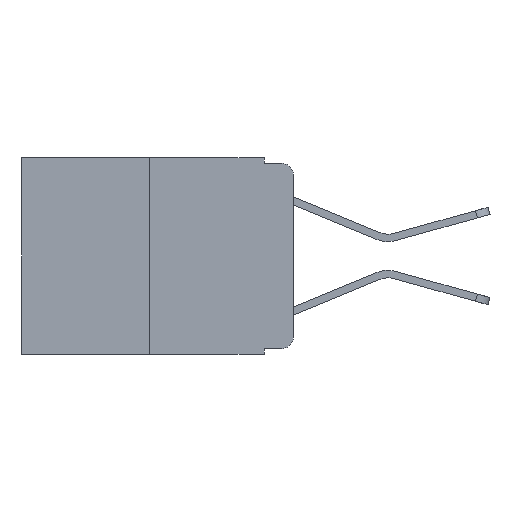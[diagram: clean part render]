
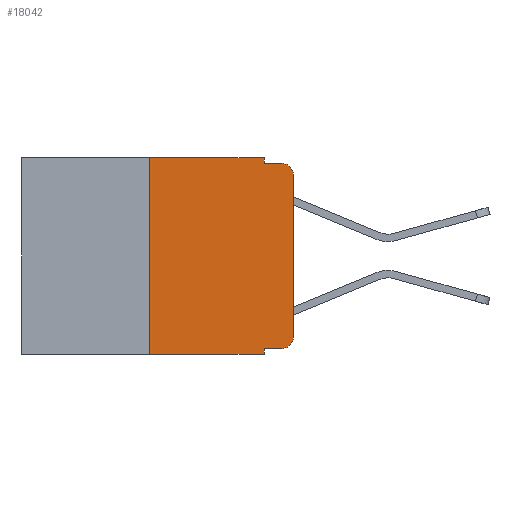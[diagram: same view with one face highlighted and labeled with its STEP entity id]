
A CAD part, left-side view. The second image highlights one B-rep face of the part: STEP entity #18042.
In plain terms, the highlighted planar face has unit normal (-1, 0, 0).
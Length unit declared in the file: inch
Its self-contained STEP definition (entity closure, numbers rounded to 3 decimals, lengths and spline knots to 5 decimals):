
#11 = AXIS2_PLACEMENT_3D ( 'NONE', #3893, #15890, #5646 ) ;
#367 = VECTOR ( 'NONE', #1647, 39.37008 ) ;
#515 = VERTEX_POINT ( 'NONE', #19281 ) ;
#532 = CARTESIAN_POINT ( 'NONE',  ( 0., 0.25, 0. ) ) ;
#1293 = CIRCLE ( 'NONE', #17704, 0.02 ) ;
#1513 = VERTEX_POINT ( 'NONE', #16426 ) ;
#1647 = DIRECTION ( 'NONE',  ( 0., 0., -1. ) ) ;
#2105 = ORIENTED_EDGE ( 'NONE', *, *, #2563, .T. ) ;
#2563 = EDGE_CURVE ( 'NONE', #11061, #7208, #16478, .T. ) ;
#2813 = VERTEX_POINT ( 'NONE', #8308 ) ;
#2828 = VERTEX_POINT ( 'NONE', #6119 ) ;
#3156 = CARTESIAN_POINT ( 'NONE',  ( 0., 0.473, 0. ) ) ;
#3276 = VECTOR ( 'NONE', #5430, 39.37008 ) ;
#3361 = VECTOR ( 'NONE', #5555, 39.37008 ) ;
#3808 = ORIENTED_EDGE ( 'NONE', *, *, #11896, .F. ) ;
#3843 = DIRECTION ( 'NONE',  ( -1., 0., 0. ) ) ;
#3893 = CARTESIAN_POINT ( 'NONE',  ( 0., 0.02, -0.313 ) ) ;
#4162 = DIRECTION ( 'NONE',  ( 0., -1., 0. ) ) ;
#4316 = EDGE_LOOP ( 'NONE', ( #2105, #18989, #14487, #5131, #14232, #5413, #20074, #3808, #8985, #16936 ) ) ;
#5041 = LINE ( 'NONE', #20484, #367 ) ;
#5057 = CARTESIAN_POINT ( 'NONE',  ( 0., 0., 0. ) ) ;
#5131 = ORIENTED_EDGE ( 'NONE', *, *, #19201, .F. ) ;
#5146 = FACE_OUTER_BOUND ( 'NONE', #4316, .T. ) ;
#5413 = ORIENTED_EDGE ( 'NONE', *, *, #20143, .F. ) ;
#5430 = DIRECTION ( 'NONE',  ( 0., -1., 0. ) ) ;
#5555 = DIRECTION ( 'NONE',  ( 0., 0., 1. ) ) ;
#5646 = DIRECTION ( 'NONE',  ( 0., 0., -1. ) ) ;
#6119 = CARTESIAN_POINT ( 'NONE',  ( 0., 0.25, -0.343 ) ) ;
#6775 = EDGE_CURVE ( 'NONE', #21434, #11061, #10975, .T. ) ;
#6824 = DIRECTION ( 'NONE',  ( 0., 0., -1. ) ) ;
#7208 = VERTEX_POINT ( 'NONE', #13591 ) ;
#7601 = CARTESIAN_POINT ( 'NONE',  ( 0., 0.051, -0.01 ) ) ;
#7661 = CARTESIAN_POINT ( 'NONE',  ( 0., 0.051, -0.333 ) ) ;
#7740 = CARTESIAN_POINT ( 'NONE',  ( 0., 0.051, -0.343 ) ) ;
#7751 = LINE ( 'NONE', #532, #20733 ) ;
#8308 = CARTESIAN_POINT ( 'NONE',  ( 0., 0.051, -0.01 ) ) ;
#8446 = LINE ( 'NONE', #17380, #3276 ) ;
#8598 = AXIS2_PLACEMENT_3D ( 'NONE', #13644, #17032, #6824 ) ;
#8691 = VECTOR ( 'NONE', #4162, 39.37008 ) ;
#8749 = VERTEX_POINT ( 'NONE', #21012 ) ;
#8985 = ORIENTED_EDGE ( 'NONE', *, *, #17056, .T. ) ;
#10399 = DIRECTION ( 'NONE',  ( 0., -1., 0. ) ) ;
#10422 = CARTESIAN_POINT ( 'NONE',  ( 0., 0., -0.313 ) ) ;
#10564 = CARTESIAN_POINT ( 'NONE',  ( 0., 0.02, -0.333 ) ) ;
#10975 = CIRCLE ( 'NONE', #11, 0.02 ) ;
#11061 = VERTEX_POINT ( 'NONE', #10422 ) ;
#11577 = CARTESIAN_POINT ( 'NONE',  ( 0., 0.051, 0. ) ) ;
#11896 = EDGE_CURVE ( 'NONE', #12143, #17716, #5041, .T. ) ;
#12143 = VERTEX_POINT ( 'NONE', #7661 ) ;
#12354 = VECTOR ( 'NONE', #21634, 39.37008 ) ;
#12663 = DIRECTION ( 'NONE',  ( 0., 0., 1. ) ) ;
#13228 = LINE ( 'NONE', #7601, #8691 ) ;
#13591 = CARTESIAN_POINT ( 'NONE',  ( 0., 0., -0.03 ) ) ;
#13644 = CARTESIAN_POINT ( 'NONE',  ( 0., 0.473, 0. ) ) ;
#13720 = EDGE_CURVE ( 'NONE', #2828, #17716, #16730, .T. ) ;
#14131 = CARTESIAN_POINT ( 'NONE',  ( 0., 0.02, -0.03 ) ) ;
#14232 = ORIENTED_EDGE ( 'NONE', *, *, #20647, .F. ) ;
#14487 = ORIENTED_EDGE ( 'NONE', *, *, #17680, .F. ) ;
#15325 = PLANE ( 'NONE',  #8598 ) ;
#15850 = DIRECTION ( 'NONE',  ( 0., 0., -1. ) ) ;
#15890 = DIRECTION ( 'NONE',  ( -1., 0., 0. ) ) ;
#16426 = CARTESIAN_POINT ( 'NONE',  ( 0., 0.02, -0.01 ) ) ;
#16478 = LINE ( 'NONE', #5057, #3361 ) ;
#16730 = LINE ( 'NONE', #22140, #17292 ) ;
#16860 = DIRECTION ( 'NONE',  ( 0., -1., 0. ) ) ;
#16936 = ORIENTED_EDGE ( 'NONE', *, *, #6775, .T. ) ;
#17032 = DIRECTION ( 'NONE',  ( 1., 0., 0. ) ) ;
#17056 = EDGE_CURVE ( 'NONE', #12143, #21434, #8446, .T. ) ;
#17292 = VECTOR ( 'NONE', #10399, 39.37008 ) ;
#17380 = CARTESIAN_POINT ( 'NONE',  ( 0., 0.051, -0.333 ) ) ;
#17680 = EDGE_CURVE ( 'NONE', #2813, #1513, #13228, .T. ) ;
#17704 = AXIS2_PLACEMENT_3D ( 'NONE', #14131, #3843, #15850 ) ;
#17716 = VERTEX_POINT ( 'NONE', #7740 ) ;
#18042 = ADVANCED_FACE ( 'NONE', ( #5146 ), #15325, .F. ) ;
#18229 = EDGE_CURVE ( 'NONE', #7208, #1513, #1293, .T. ) ;
#18989 = ORIENTED_EDGE ( 'NONE', *, *, #18229, .T. ) ;
#19174 = LINE ( 'NONE', #3156, #22002 ) ;
#19201 = EDGE_CURVE ( 'NONE', #8749, #2813, #21266, .T. ) ;
#19281 = CARTESIAN_POINT ( 'NONE',  ( 0., 0.25, 0. ) ) ;
#20074 = ORIENTED_EDGE ( 'NONE', *, *, #13720, .T. ) ;
#20143 = EDGE_CURVE ( 'NONE', #2828, #515, #7751, .T. ) ;
#20484 = CARTESIAN_POINT ( 'NONE',  ( 0., 0.051, 0. ) ) ;
#20647 = EDGE_CURVE ( 'NONE', #515, #8749, #19174, .T. ) ;
#20733 = VECTOR ( 'NONE', #12663, 39.37008 ) ;
#21012 = CARTESIAN_POINT ( 'NONE',  ( 0., 0.051, 0. ) ) ;
#21266 = LINE ( 'NONE', #11577, #12354 ) ;
#21434 = VERTEX_POINT ( 'NONE', #10564 ) ;
#21634 = DIRECTION ( 'NONE',  ( 0., 0., -1. ) ) ;
#22002 = VECTOR ( 'NONE', #16860, 39.37008 ) ;
#22140 = CARTESIAN_POINT ( 'NONE',  ( 0., 0.473, -0.343 ) ) ;
